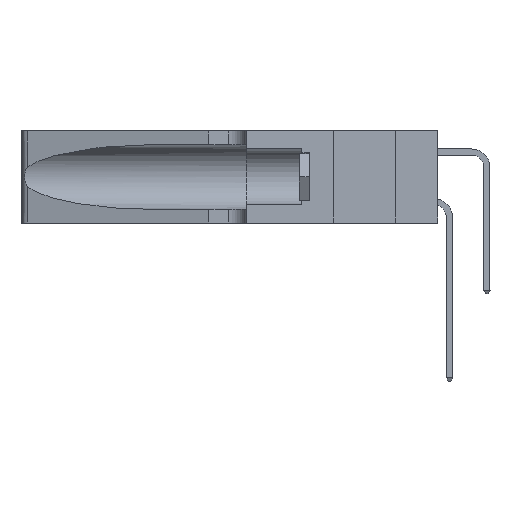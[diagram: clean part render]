
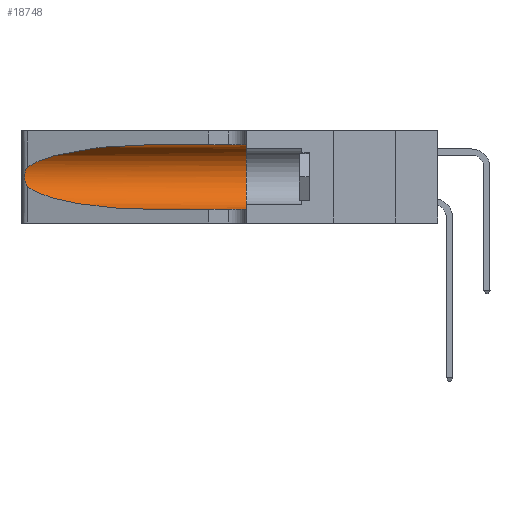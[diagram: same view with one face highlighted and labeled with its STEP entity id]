
A CAD part, left-side view. The second image highlights one B-rep face of the part: STEP entity #18748.
In plain terms, the highlighted cylindrical face has radius 3.308 mm (diameter 6.617 mm), a partial arc.
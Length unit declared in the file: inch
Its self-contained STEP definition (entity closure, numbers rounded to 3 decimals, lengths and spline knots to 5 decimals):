
#491 = CARTESIAN_POINT ( 'NONE',  ( 0.1305, 0.72297, 0.05475 ) ) ;
#964 = DIRECTION ( 'NONE',  ( 0., -1., 0. ) ) ;
#1397 = CARTESIAN_POINT ( 'NONE',  ( 0.25854, 1.2359, 0.20912 ) ) ;
#1819 = CARTESIAN_POINT ( 'NONE',  ( 0.25639, 1.23184, 0.21858 ) ) ;
#4033 = CARTESIAN_POINT ( 'NONE',  ( 0.25487, 1.22718, 0.14631 ) ) ;
#4102 = CARTESIAN_POINT ( 'NONE',  ( 0.25555, 1.22994, 0.2215 ) ) ;
#4149 = CARTESIAN_POINT ( 'NONE',  ( 0.2373, 1.15595, 0.28018 ) ) ;
#4339 = CYLINDRICAL_SURFACE ( 'NONE', #10324, 0.13025 ) ;
#4357 = CARTESIAN_POINT ( 'NONE',  ( 0.25487, 1.22718, 0.22369 ) ) ;
#6007 =( BOUNDED_CURVE ( )  B_SPLINE_CURVE ( 3, ( #18493, #18712, #4149, #4357 ),
 .UNSPECIFIED., .F., .T. ) 
 B_SPLINE_CURVE_WITH_KNOTS ( ( 4, 4 ),
 ( 1.5708, 2.84003 ),
 .UNSPECIFIED. ) 
 CURVE ( )  GEOMETRIC_REPRESENTATION_ITEM ( )  RATIONAL_B_SPLINE_CURVE ( ( 1., 0.87, 0.87, 1. ) ) 
 REPRESENTATION_ITEM ( '' )  );
#7050 = VERTEX_POINT ( 'NONE', #491 ) ;
#7262 = DIRECTION ( 'NONE',  ( 0., 0., -1. ) ) ;
#7884 = ORIENTED_EDGE ( 'NONE', *, *, #30374, .F. ) ;
#7955 = VERTEX_POINT ( 'NONE', #17462 ) ;
#8109 = FACE_OUTER_BOUND ( 'NONE', #16549, .T. ) ;
#8748 = CARTESIAN_POINT ( 'NONE',  ( 0.25487, 1.22718, 0.22369 ) ) ;
#8852 = ORIENTED_EDGE ( 'NONE', *, *, #25040, .T. ) ;
#8886 = CARTESIAN_POINT ( 'NONE',  ( 0.18966, 0.96281, 0.05475 ) ) ;
#8950 = EDGE_CURVE ( 'NONE', #21899, #26423, #6007, .T. ) ;
#9368 = CARTESIAN_POINT ( 'NONE',  ( 0.26075, 1.23896, 0.178 ) ) ;
#10324 = AXIS2_PLACEMENT_3D ( 'NONE', #30691, #28797, #7262 ) ;
#10805 = CIRCLE ( 'NONE', #22925, 0.13025 ) ;
#11449 = CARTESIAN_POINT ( 'NONE',  ( 0.25789, 1.23486, 0.15765 ) ) ;
#11767 = CARTESIAN_POINT ( 'NONE',  ( 0.26075, 1.23896, 0.19203 ) ) ;
#12283 = ORIENTED_EDGE ( 'NONE', *, *, #26298, .T. ) ;
#14160 = CARTESIAN_POINT ( 'NONE',  ( 0.25856, 1.23593, 0.16098 ) ) ;
#15509 = VERTEX_POINT ( 'NONE', #27714 ) ;
#15525 = CARTESIAN_POINT ( 'NONE',  ( 0.25487, 1.22718, 0.14631 ) ) ;
#15989 = CARTESIAN_POINT ( 'NONE',  ( 0.2373, 1.15595, 0.08982 ) ) ;
#16260 = CARTESIAN_POINT ( 'NONE',  ( 0.26017, 1.23833, 0.17102 ) ) ;
#16459 = CARTESIAN_POINT ( 'NONE',  ( 0.25487, 1.22718, 0.14631 ) ) ;
#16549 = EDGE_LOOP ( 'NONE', ( #26942, #12283, #29369, #8852, #7884, #17810 ) ) ;
#16563 = CARTESIAN_POINT ( 'NONE',  ( 0.25639, 1.23186, 0.15144 ) ) ;
#17462 = CARTESIAN_POINT ( 'NONE',  ( 0.1305, 0.35, 0.31525 ) ) ;
#17685 = CARTESIAN_POINT ( 'NONE',  ( 0.1305, 1.61858, 0.05475 ) ) ;
#17810 = ORIENTED_EDGE ( 'NONE', *, *, #24944, .F. ) ;
#18123 = CARTESIAN_POINT ( 'NONE',  ( 0.26018, 1.23835, 0.19895 ) ) ;
#18493 = CARTESIAN_POINT ( 'NONE',  ( 0.1305, 0.72297, 0.31525 ) ) ;
#18712 = CARTESIAN_POINT ( 'NONE',  ( 0.18966, 0.96281, 0.31525 ) ) ;
#18748 = ADVANCED_FACE ( 'NONE', ( #8109 ), #4339, .F. ) ;
#19552 = VECTOR ( 'NONE', #964, 39.37008 ) ;
#20703 = EDGE_CURVE ( 'NONE', #21794, #7050, #28329, .T. ) ;
#21794 = VERTEX_POINT ( 'NONE', #15525 ) ;
#21899 = VERTEX_POINT ( 'NONE', #30641 ) ;
#22159 = LINE ( 'NONE', #29291, #27079 ) ;
#22693 = DIRECTION ( 'NONE',  ( 0., 1., 0. ) ) ;
#22925 = AXIS2_PLACEMENT_3D ( 'NONE', #25230, #22693, #25122 ) ;
#24321 = DIRECTION ( 'NONE',  ( 0., -1., 0. ) ) ;
#24944 = EDGE_CURVE ( 'NONE', #21899, #7955, #22159, .T. ) ;
#25040 = EDGE_CURVE ( 'NONE', #7050, #15509, #28615, .T. ) ;
#25122 = DIRECTION ( 'NONE',  ( 0., 0., 1. ) ) ;
#25230 = CARTESIAN_POINT ( 'NONE',  ( 0.1305, 0.35, 0.185 ) ) ;
#26298 = EDGE_CURVE ( 'NONE', #26423, #21794, #26937, .T. ) ;
#26423 = VERTEX_POINT ( 'NONE', #28457 ) ;
#26937 = B_SPLINE_CURVE_WITH_KNOTS ( 'NONE', 3,
 ( #8748, #4102, #1819, #27719, #1397, #18123, #11767, #9368, #16260, #14160, #11449, #16563, #30870, #16459 ),
 .UNSPECIFIED., .F., .F.,
 ( 4, 2, 2, 2, 2, 2, 4 ),
 ( 0., 0.00027, 0.00053, 0.00107, 0.0016, 0.00187, 0.00214 ),
 .UNSPECIFIED. ) ;
#26942 = ORIENTED_EDGE ( 'NONE', *, *, #8950, .T. ) ;
#27079 = VECTOR ( 'NONE', #24321, 39.37008 ) ;
#27714 = CARTESIAN_POINT ( 'NONE',  ( 0.1305, 0.35, 0.05475 ) ) ;
#27719 = CARTESIAN_POINT ( 'NONE',  ( 0.25787, 1.23484, 0.2124 ) ) ;
#27858 = CARTESIAN_POINT ( 'NONE',  ( 0.1305, 0.72297, 0.05475 ) ) ;
#28329 =( BOUNDED_CURVE ( )  B_SPLINE_CURVE ( 3, ( #4033, #15989, #8886, #27858 ),
 .UNSPECIFIED., .F., .T. ) 
 B_SPLINE_CURVE_WITH_KNOTS ( ( 4, 4 ),
 ( 3.44316, 4.71239 ),
 .UNSPECIFIED. ) 
 CURVE ( )  GEOMETRIC_REPRESENTATION_ITEM ( )  RATIONAL_B_SPLINE_CURVE ( ( 1., 0.87, 0.87, 1. ) ) 
 REPRESENTATION_ITEM ( '' )  );
#28457 = CARTESIAN_POINT ( 'NONE',  ( 0.25487, 1.22718, 0.22369 ) ) ;
#28615 = LINE ( 'NONE', #17685, #19552 ) ;
#28797 = DIRECTION ( 'NONE',  ( 0., -1., 0. ) ) ;
#29291 = CARTESIAN_POINT ( 'NONE',  ( 0.1305, 1.61858, 0.31525 ) ) ;
#29369 = ORIENTED_EDGE ( 'NONE', *, *, #20703, .T. ) ;
#30374 = EDGE_CURVE ( 'NONE', #7955, #15509, #10805, .T. ) ;
#30641 = CARTESIAN_POINT ( 'NONE',  ( 0.1305, 0.72297, 0.31525 ) ) ;
#30691 = CARTESIAN_POINT ( 'NONE',  ( 0.1305, 1.61858, 0.185 ) ) ;
#30870 = CARTESIAN_POINT ( 'NONE',  ( 0.25555, 1.22993, 0.14849 ) ) ;
